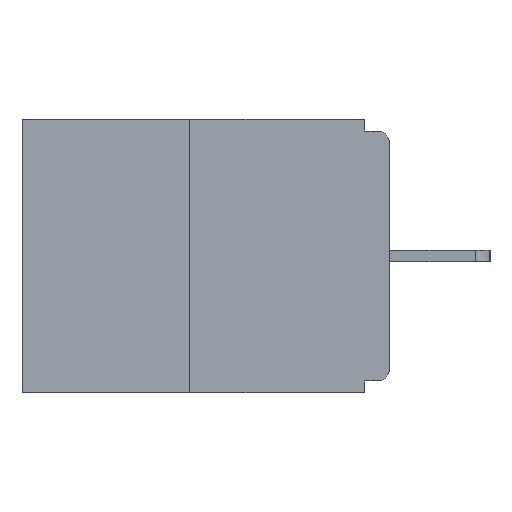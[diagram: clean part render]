
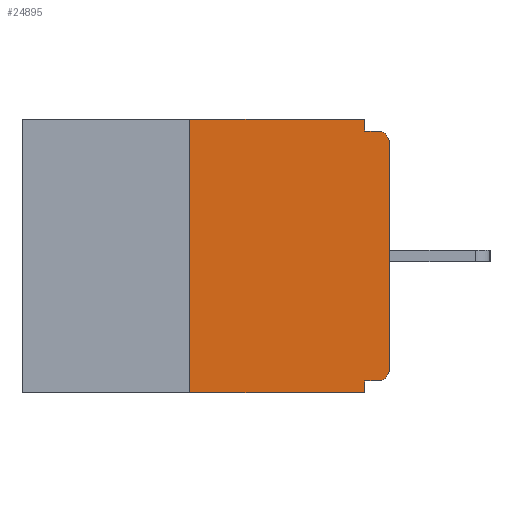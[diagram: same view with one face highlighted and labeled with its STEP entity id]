
A CAD part, left-side view. The second image highlights one B-rep face of the part: STEP entity #24895.
In plain terms, the highlighted planar face has unit normal (-1, 0, 0).
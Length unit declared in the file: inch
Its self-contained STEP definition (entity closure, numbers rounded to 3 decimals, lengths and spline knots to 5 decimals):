
#44 = CARTESIAN_POINT ( 'NONE',  ( 0., 0.46, 0. ) ) ;
#410 = DIRECTION ( 'NONE',  ( 0., 0., -1. ) ) ;
#460 = LINE ( 'NONE', #10568, #26499 ) ;
#472 = VECTOR ( 'NONE', #12350, 39.37008 ) ;
#670 = CARTESIAN_POINT ( 'NONE',  ( 0., 0.031, 0. ) ) ;
#1341 = CARTESIAN_POINT ( 'NONE',  ( 0., 0.031, -0.015 ) ) ;
#1687 = CIRCLE ( 'NONE', #12852, 0.015 ) ;
#1912 = ORIENTED_EDGE ( 'NONE', *, *, #10426, .F. ) ;
#2232 = VECTOR ( 'NONE', #3241, 39.37008 ) ;
#2273 = EDGE_LOOP ( 'NONE', ( #16927, #12344, #5494, #10577, #1912, #16398, #18371, #18021, #7515, #17091 ) ) ;
#2297 = DIRECTION ( 'NONE',  ( 0., 0., -1. ) ) ;
#2556 = CARTESIAN_POINT ( 'NONE',  ( 0., 0.46, 0. ) ) ;
#2660 = VERTEX_POINT ( 'NONE', #4100 ) ;
#2736 = VERTEX_POINT ( 'NONE', #22854 ) ;
#3241 = DIRECTION ( 'NONE',  ( 0., -1., 0. ) ) ;
#3289 = VERTEX_POINT ( 'NONE', #17821 ) ;
#3300 = CARTESIAN_POINT ( 'NONE',  ( 0., 0.25, 0. ) ) ;
#4100 = CARTESIAN_POINT ( 'NONE',  ( 0., 0.015, -0.328 ) ) ;
#4917 = VERTEX_POINT ( 'NONE', #8350 ) ;
#5494 = ORIENTED_EDGE ( 'NONE', *, *, #25456, .T. ) ;
#5980 = VERTEX_POINT ( 'NONE', #25738 ) ;
#6072 = CARTESIAN_POINT ( 'NONE',  ( 0., 0.015, -0.313 ) ) ;
#6718 = DIRECTION ( 'NONE',  ( 0., 0., -1. ) ) ;
#7334 = DIRECTION ( 'NONE',  ( 0., 0., 1. ) ) ;
#7490 = EDGE_CURVE ( 'NONE', #2660, #3289, #18044, .T. ) ;
#7515 = ORIENTED_EDGE ( 'NONE', *, *, #25754, .F. ) ;
#8350 = CARTESIAN_POINT ( 'NONE',  ( 0., 0.031, -0.343 ) ) ;
#8545 = CARTESIAN_POINT ( 'NONE',  ( 0., 0.031, -0.343 ) ) ;
#8599 = CARTESIAN_POINT ( 'NONE',  ( 0., 0.031, 0. ) ) ;
#8739 = DIRECTION ( 'NONE',  ( -1., 0., 0. ) ) ;
#8762 = VECTOR ( 'NONE', #24459, 39.37008 ) ;
#9055 = AXIS2_PLACEMENT_3D ( 'NONE', #2556, #21176, #20921 ) ;
#9171 = VECTOR ( 'NONE', #21356, 39.37008 ) ;
#9346 = CARTESIAN_POINT ( 'NONE',  ( 0., 0.46, -0.343 ) ) ;
#9442 = CARTESIAN_POINT ( 'NONE',  ( 0., 0., -0.328 ) ) ;
#9478 = DIRECTION ( 'NONE',  ( 0., -1., 0. ) ) ;
#9717 = CARTESIAN_POINT ( 'NONE',  ( 0., 0., -0.03 ) ) ;
#10013 = VERTEX_POINT ( 'NONE', #3300 ) ;
#10426 = EDGE_CURVE ( 'NONE', #2660, #2736, #23516, .T. ) ;
#10568 = CARTESIAN_POINT ( 'NONE',  ( 0., 0.25, 0. ) ) ;
#10577 = ORIENTED_EDGE ( 'NONE', *, *, #25115, .F. ) ;
#10584 = VERTEX_POINT ( 'NONE', #9717 ) ;
#11426 = EDGE_CURVE ( 'NONE', #10013, #19803, #18130, .T. ) ;
#11458 = CARTESIAN_POINT ( 'NONE',  ( 0., 0., -0.015 ) ) ;
#11482 = CARTESIAN_POINT ( 'NONE',  ( 0., 0.015, -0.015 ) ) ;
#11702 = VECTOR ( 'NONE', #9478, 39.37008 ) ;
#12344 = ORIENTED_EDGE ( 'NONE', *, *, #13917, .F. ) ;
#12350 = DIRECTION ( 'NONE',  ( 0., 0., -1. ) ) ;
#12852 = AXIS2_PLACEMENT_3D ( 'NONE', #21173, #8739, #6718 ) ;
#13409 = LINE ( 'NONE', #15447, #23152 ) ;
#13917 = EDGE_CURVE ( 'NONE', #5980, #10013, #460, .T. ) ;
#14467 = DIRECTION ( 'NONE',  ( -1., 0., 0. ) ) ;
#15226 = EDGE_CURVE ( 'NONE', #3289, #10584, #13409, .T. ) ;
#15447 = CARTESIAN_POINT ( 'NONE',  ( 0., 0., 0. ) ) ;
#16398 = ORIENTED_EDGE ( 'NONE', *, *, #7490, .T. ) ;
#16598 = FACE_OUTER_BOUND ( 'NONE', #2273, .T. ) ;
#16927 = ORIENTED_EDGE ( 'NONE', *, *, #11426, .F. ) ;
#17091 = ORIENTED_EDGE ( 'NONE', *, *, #19774, .F. ) ;
#17821 = CARTESIAN_POINT ( 'NONE',  ( 0., 0., -0.313 ) ) ;
#18021 = ORIENTED_EDGE ( 'NONE', *, *, #21096, .T. ) ;
#18044 = CIRCLE ( 'NONE', #21495, 0.015 ) ;
#18130 = LINE ( 'NONE', #44, #8762 ) ;
#18371 = ORIENTED_EDGE ( 'NONE', *, *, #15226, .T. ) ;
#18422 = LINE ( 'NONE', #8545, #472 ) ;
#19761 = LINE ( 'NONE', #9346, #11702 ) ;
#19774 = EDGE_CURVE ( 'NONE', #19803, #19928, #20771, .T. ) ;
#19803 = VERTEX_POINT ( 'NONE', #670 ) ;
#19928 = VERTEX_POINT ( 'NONE', #1341 ) ;
#20771 = LINE ( 'NONE', #8599, #25479 ) ;
#20921 = DIRECTION ( 'NONE',  ( 0., 0., -1. ) ) ;
#21096 = EDGE_CURVE ( 'NONE', #10584, #24538, #1687, .T. ) ;
#21173 = CARTESIAN_POINT ( 'NONE',  ( 0., 0.015, -0.03 ) ) ;
#21176 = DIRECTION ( 'NONE',  ( 1., 0., 0. ) ) ;
#21187 = LINE ( 'NONE', #11458, #2232 ) ;
#21356 = DIRECTION ( 'NONE',  ( 0., 1., 0. ) ) ;
#21495 = AXIS2_PLACEMENT_3D ( 'NONE', #6072, #14467, #410 ) ;
#22854 = CARTESIAN_POINT ( 'NONE',  ( 0., 0.031, -0.328 ) ) ;
#23152 = VECTOR ( 'NONE', #7334, 39.37008 ) ;
#23516 = LINE ( 'NONE', #9442, #9171 ) ;
#24459 = DIRECTION ( 'NONE',  ( 0., -1., 0. ) ) ;
#24538 = VERTEX_POINT ( 'NONE', #11482 ) ;
#24895 = ADVANCED_FACE ( 'NONE', ( #16598 ), #25070, .F. ) ;
#25070 = PLANE ( 'NONE',  #9055 ) ;
#25115 = EDGE_CURVE ( 'NONE', #2736, #4917, #18422, .T. ) ;
#25456 = EDGE_CURVE ( 'NONE', #5980, #4917, #19761, .T. ) ;
#25479 = VECTOR ( 'NONE', #2297, 39.37008 ) ;
#25738 = CARTESIAN_POINT ( 'NONE',  ( 0., 0.25, -0.343 ) ) ;
#25754 = EDGE_CURVE ( 'NONE', #19928, #24538, #21187, .T. ) ;
#26499 = VECTOR ( 'NONE', #26636, 39.37008 ) ;
#26636 = DIRECTION ( 'NONE',  ( 0., 0., 1. ) ) ;
